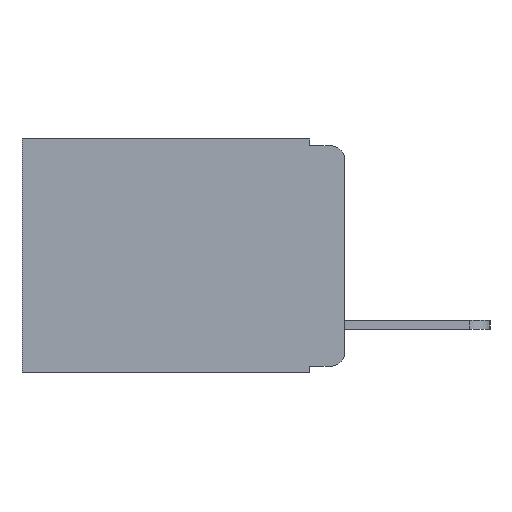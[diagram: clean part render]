
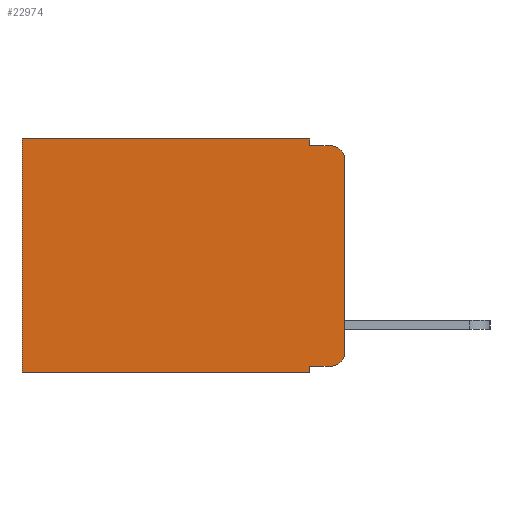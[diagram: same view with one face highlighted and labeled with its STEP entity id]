
A CAD part, left-side view. The second image highlights one B-rep face of the part: STEP entity #22974.
In plain terms, the highlighted planar face has unit normal (-1, 0, 0).
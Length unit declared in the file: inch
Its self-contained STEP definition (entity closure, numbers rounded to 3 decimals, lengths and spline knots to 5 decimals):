
#64 = LINE ( 'NONE', #20917, #704 ) ;
#154 = VERTEX_POINT ( 'NONE', #4094 ) ;
#585 = EDGE_LOOP ( 'NONE', ( #18756, #6154, #4502, #3835, #11529, #21073, #790, #1969, #10610, #9594 ) ) ;
#704 = VECTOR ( 'NONE', #23674, 39.37008 ) ;
#790 = ORIENTED_EDGE ( 'NONE', *, *, #5185, .F. ) ;
#1102 = VERTEX_POINT ( 'NONE', #5019 ) ;
#1138 = LINE ( 'NONE', #18231, #21012 ) ;
#1672 = LINE ( 'NONE', #16618, #11679 ) ;
#1969 = ORIENTED_EDGE ( 'NONE', *, *, #12789, .F. ) ;
#1997 = AXIS2_PLACEMENT_3D ( 'NONE', #22234, #11077, #24050 ) ;
#2108 = FACE_OUTER_BOUND ( 'NONE', #585, .T. ) ;
#2687 = DIRECTION ( 'NONE',  ( 0., 0., -1. ) ) ;
#2901 = CARTESIAN_POINT ( 'NONE',  ( 0.298, 0.051, -0.01 ) ) ;
#3079 = CARTESIAN_POINT ( 'NONE',  ( 0.298, 0.051, -0.333 ) ) ;
#3343 = VECTOR ( 'NONE', #22215, 39.37008 ) ;
#3835 = ORIENTED_EDGE ( 'NONE', *, *, #21240, .F. ) ;
#3934 = LINE ( 'NONE', #10684, #13816 ) ;
#4094 = CARTESIAN_POINT ( 'NONE',  ( 0.298, 0., -0.03 ) ) ;
#4127 = VERTEX_POINT ( 'NONE', #16249 ) ;
#4167 = CARTESIAN_POINT ( 'NONE',  ( 0.298, 0.051, 0. ) ) ;
#4502 = ORIENTED_EDGE ( 'NONE', *, *, #8312, .F. ) ;
#4830 = EDGE_CURVE ( 'NONE', #12055, #1102, #3934, .T. ) ;
#5019 = CARTESIAN_POINT ( 'NONE',  ( 0.298, 0.473, 0. ) ) ;
#5185 = EDGE_CURVE ( 'NONE', #4127, #6858, #1672, .T. ) ;
#5201 = CARTESIAN_POINT ( 'NONE',  ( 0.298, 0.02, -0.03 ) ) ;
#5332 = VERTEX_POINT ( 'NONE', #13979 ) ;
#5566 = CIRCLE ( 'NONE', #8985, 0.02 ) ;
#5831 = DIRECTION ( 'NONE',  ( 0., 0., -1. ) ) ;
#6009 = DIRECTION ( 'NONE',  ( 0., 1., 0. ) ) ;
#6154 = ORIENTED_EDGE ( 'NONE', *, *, #15487, .T. ) ;
#6247 = CARTESIAN_POINT ( 'NONE',  ( 0.298, 0., -0.313 ) ) ;
#6851 = CARTESIAN_POINT ( 'NONE',  ( 0.298, 0.473, -0.343 ) ) ;
#6858 = VERTEX_POINT ( 'NONE', #6851 ) ;
#6996 = DIRECTION ( 'NONE',  ( 0., 0., -1. ) ) ;
#7142 = PLANE ( 'NONE',  #1997 ) ;
#7291 = EDGE_CURVE ( 'NONE', #154, #19360, #16210, .T. ) ;
#8312 = EDGE_CURVE ( 'NONE', #20429, #18071, #16731, .T. ) ;
#8442 = CARTESIAN_POINT ( 'NONE',  ( 0.298, 0., 0. ) ) ;
#8985 = AXIS2_PLACEMENT_3D ( 'NONE', #5201, #20641, #5831 ) ;
#9043 = DIRECTION ( 'NONE',  ( 0., 1., 0. ) ) ;
#9594 = ORIENTED_EDGE ( 'NONE', *, *, #19089, .T. ) ;
#9759 = CIRCLE ( 'NONE', #17666, 0.02 ) ;
#10610 = ORIENTED_EDGE ( 'NONE', *, *, #16332, .T. ) ;
#10684 = CARTESIAN_POINT ( 'NONE',  ( 0.298, 0., 0. ) ) ;
#11077 = DIRECTION ( 'NONE',  ( 1., 0., 0. ) ) ;
#11529 = ORIENTED_EDGE ( 'NONE', *, *, #4830, .T. ) ;
#11679 = VECTOR ( 'NONE', #6009, 39.37008 ) ;
#12055 = VERTEX_POINT ( 'NONE', #20987 ) ;
#12789 = EDGE_CURVE ( 'NONE', #20485, #4127, #20804, .T. ) ;
#13816 = VECTOR ( 'NONE', #9043, 39.37008 ) ;
#13853 = LINE ( 'NONE', #16977, #3343 ) ;
#13979 = CARTESIAN_POINT ( 'NONE',  ( 0.298, 0.02, -0.333 ) ) ;
#13991 = CARTESIAN_POINT ( 'NONE',  ( 0.298, 0.02, -0.01 ) ) ;
#14603 = DIRECTION ( 'NONE',  ( 0., 0., -1. ) ) ;
#14908 = EDGE_CURVE ( 'NONE', #1102, #6858, #1138, .T. ) ;
#15487 = EDGE_CURVE ( 'NONE', #154, #18071, #5566, .T. ) ;
#15611 = CARTESIAN_POINT ( 'NONE',  ( 0.298, 0.051, -0.01 ) ) ;
#15874 = VECTOR ( 'NONE', #2687, 39.37008 ) ;
#16179 = DIRECTION ( 'NONE',  ( 0., 0., -1. ) ) ;
#16210 = LINE ( 'NONE', #8442, #21743 ) ;
#16249 = CARTESIAN_POINT ( 'NONE',  ( 0.298, 0.051, -0.343 ) ) ;
#16277 = CARTESIAN_POINT ( 'NONE',  ( 0.298, 0.02, -0.313 ) ) ;
#16300 = DIRECTION ( 'NONE',  ( -1., 0., 0. ) ) ;
#16332 = EDGE_CURVE ( 'NONE', #20485, #5332, #13853, .T. ) ;
#16618 = CARTESIAN_POINT ( 'NONE',  ( 0.298, 0., -0.343 ) ) ;
#16731 = LINE ( 'NONE', #15611, #21099 ) ;
#16838 = DIRECTION ( 'NONE',  ( 0., -1., 0. ) ) ;
#16977 = CARTESIAN_POINT ( 'NONE',  ( 0.298, 0.051, -0.333 ) ) ;
#17666 = AXIS2_PLACEMENT_3D ( 'NONE', #16277, #16300, #16179 ) ;
#18071 = VERTEX_POINT ( 'NONE', #13991 ) ;
#18231 = CARTESIAN_POINT ( 'NONE',  ( 0.298, 0.473, 0. ) ) ;
#18756 = ORIENTED_EDGE ( 'NONE', *, *, #7291, .F. ) ;
#19089 = EDGE_CURVE ( 'NONE', #5332, #19360, #9759, .T. ) ;
#19360 = VERTEX_POINT ( 'NONE', #6247 ) ;
#20429 = VERTEX_POINT ( 'NONE', #2901 ) ;
#20485 = VERTEX_POINT ( 'NONE', #3079 ) ;
#20641 = DIRECTION ( 'NONE',  ( -1., 0., 0. ) ) ;
#20804 = LINE ( 'NONE', #4167, #15874 ) ;
#20917 = CARTESIAN_POINT ( 'NONE',  ( 0.298, 0.051, 0. ) ) ;
#20987 = CARTESIAN_POINT ( 'NONE',  ( 0.298, 0.051, 0. ) ) ;
#21012 = VECTOR ( 'NONE', #14603, 39.37008 ) ;
#21073 = ORIENTED_EDGE ( 'NONE', *, *, #14908, .T. ) ;
#21099 = VECTOR ( 'NONE', #16838, 39.37008 ) ;
#21240 = EDGE_CURVE ( 'NONE', #12055, #20429, #64, .T. ) ;
#21743 = VECTOR ( 'NONE', #6996, 39.37008 ) ;
#22215 = DIRECTION ( 'NONE',  ( 0., -1., 0. ) ) ;
#22234 = CARTESIAN_POINT ( 'NONE',  ( 0.298, 0., 0. ) ) ;
#22974 = ADVANCED_FACE ( 'NONE', ( #2108 ), #7142, .F. ) ;
#23674 = DIRECTION ( 'NONE',  ( 0., 0., -1. ) ) ;
#24050 = DIRECTION ( 'NONE',  ( 0., 0., -1. ) ) ;
